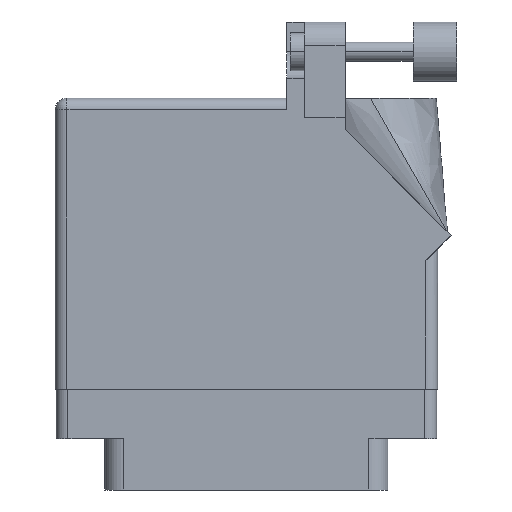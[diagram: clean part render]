
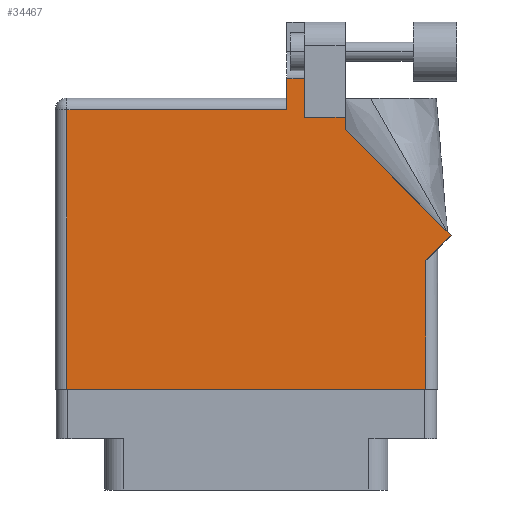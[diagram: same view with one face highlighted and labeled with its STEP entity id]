
A CAD part, front view. The second image highlights one B-rep face of the part: STEP entity #34467.
In plain terms, the highlighted face is planar.
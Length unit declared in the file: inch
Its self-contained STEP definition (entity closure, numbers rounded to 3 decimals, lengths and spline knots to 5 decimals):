
#255 = VECTOR ( 'NONE', #7287, 39.37008 ) ;
#1257 = VERTEX_POINT ( 'NONE', #19665 ) ;
#1385 = VECTOR ( 'NONE', #22672, 39.37008 ) ;
#1567 = LINE ( 'NONE', #26114, #7909 ) ;
#1798 = VERTEX_POINT ( 'NONE', #22263 ) ;
#2191 = CARTESIAN_POINT ( 'NONE',  ( 1.524, 1.36442, 0. ) ) ;
#2222 = LINE ( 'NONE', #28144, #1385 ) ;
#2418 = LINE ( 'NONE', #13033, #13001 ) ;
#2590 = VECTOR ( 'NONE', #5497, 39.37008 ) ;
#2717 = CARTESIAN_POINT ( 'NONE',  ( 1.948, 0.737, 0. ) ) ;
#2965 = VERTEX_POINT ( 'NONE', #5705 ) ;
#3114 = AXIS2_PLACEMENT_3D ( 'NONE', #13466, #18957, #32597 ) ;
#3211 = VERTEX_POINT ( 'NONE', #22888 ) ;
#4034 = DIRECTION ( 'NONE',  ( 0., 1., 0. ) ) ;
#5241 = EDGE_CURVE ( 'NONE', #28730, #2965, #20083, .T. ) ;
#5497 = DIRECTION ( 'NONE',  ( 1., 0., 0. ) ) ;
#5705 = CARTESIAN_POINT ( 'NONE',  ( 1.948, 0., 0. ) ) ;
#6089 = ORIENTED_EDGE ( 'NONE', *, *, #28696, .T. ) ;
#7287 = DIRECTION ( 'NONE',  ( 0., 1., 0. ) ) ;
#7909 = VECTOR ( 'NONE', #4034, 39.37008 ) ;
#8691 = EDGE_CURVE ( 'NONE', #3211, #1798, #18629, .T. ) ;
#8774 = DIRECTION ( 'NONE',  ( -1., 0., 0. ) ) ;
#8823 = EDGE_CURVE ( 'NONE', #13639, #29951, #1567, .T. ) ;
#9068 = ORIENTED_EDGE ( 'NONE', *, *, #5241, .T. ) ;
#9640 = ORIENTED_EDGE ( 'NONE', *, *, #9676, .T. ) ;
#9676 = EDGE_CURVE ( 'NONE', #1798, #28730, #2418, .T. ) ;
#10128 = EDGE_LOOP ( 'NONE', ( #23997, #32514, #20577, #15346, #9640, #9068, #22942, #32574, #21811, #6089, #27117 ) ) ;
#10708 = EDGE_CURVE ( 'NONE', #15570, #1257, #27729, .T. ) ;
#10904 = LINE ( 'NONE', #2191, #255 ) ;
#12149 = DIRECTION ( 'NONE',  ( -0.707, 0.707, 0. ) ) ;
#12798 = VECTOR ( 'NONE', #23317, 39.37008 ) ;
#13001 = VECTOR ( 'NONE', #32050, 39.37008 ) ;
#13033 = CARTESIAN_POINT ( 'NONE',  ( 0.062, 0., 0. ) ) ;
#13466 = CARTESIAN_POINT ( 'NONE',  ( 0., 1.53, 0. ) ) ;
#13639 = VERTEX_POINT ( 'NONE', #15105 ) ;
#14766 = CARTESIAN_POINT ( 'NONE',  ( 1.311, 1.6315, 0. ) ) ;
#14802 = CARTESIAN_POINT ( 'NONE',  ( 1.217, 1.53, 0. ) ) ;
#15105 = CARTESIAN_POINT ( 'NONE',  ( 1.311, 1.43, 0. ) ) ;
#15196 = EDGE_CURVE ( 'NONE', #29951, #26422, #27472, .T. ) ;
#15304 = CARTESIAN_POINT ( 'NONE',  ( 1.524, 1.43, 0. ) ) ;
#15346 = ORIENTED_EDGE ( 'NONE', *, *, #8691, .T. ) ;
#15507 = CARTESIAN_POINT ( 'NONE',  ( 0.062, 0., 0. ) ) ;
#15568 = EDGE_CURVE ( 'NONE', #33838, #13639, #29914, .T. ) ;
#15570 = VERTEX_POINT ( 'NONE', #18388 ) ;
#16088 = EDGE_CURVE ( 'NONE', #24751, #15570, #2222, .T. ) ;
#16403 = CARTESIAN_POINT ( 'NONE',  ( 1.64177, 1.6315, 0. ) ) ;
#16776 = VECTOR ( 'NONE', #30076, 39.37008 ) ;
#17356 = EDGE_CURVE ( 'NONE', #26422, #3211, #29828, .T. ) ;
#17864 = VECTOR ( 'NONE', #18813, 39.37008 ) ;
#18223 = EDGE_CURVE ( 'NONE', #2965, #24751, #25562, .T. ) ;
#18388 = CARTESIAN_POINT ( 'NONE',  ( 2.08071, 0.80771, 0. ) ) ;
#18629 = LINE ( 'NONE', #25144, #26313 ) ;
#18813 = DIRECTION ( 'NONE',  ( 0., 1., 0. ) ) ;
#18957 = DIRECTION ( 'NONE',  ( 0., 0., -1. ) ) ;
#19609 = VECTOR ( 'NONE', #12149, 39.37008 ) ;
#19665 = CARTESIAN_POINT ( 'NONE',  ( 1.524, 1.36442, 0. ) ) ;
#20083 = LINE ( 'NONE', #29794, #2590 ) ;
#20310 = CARTESIAN_POINT ( 'NONE',  ( 1.524, 1.43, 0. ) ) ;
#20577 = ORIENTED_EDGE ( 'NONE', *, *, #17356, .T. ) ;
#21139 = FACE_OUTER_BOUND ( 'NONE', #10128, .T. ) ;
#21811 = ORIENTED_EDGE ( 'NONE', *, *, #10708, .T. ) ;
#22263 = CARTESIAN_POINT ( 'NONE',  ( 0.062, 1.468, 0. ) ) ;
#22672 = DIRECTION ( 'NONE',  ( 0.707, 0.707, 0. ) ) ;
#22724 = VECTOR ( 'NONE', #34649, 39.37008 ) ;
#22888 = CARTESIAN_POINT ( 'NONE',  ( 1.217, 1.468, 0. ) ) ;
#22942 = ORIENTED_EDGE ( 'NONE', *, *, #18223, .T. ) ;
#23317 = DIRECTION ( 'NONE',  ( 0., -1., 0. ) ) ;
#23997 = ORIENTED_EDGE ( 'NONE', *, *, #8823, .T. ) ;
#24751 = VERTEX_POINT ( 'NONE', #35174 ) ;
#25144 = CARTESIAN_POINT ( 'NONE',  ( 0., 1.468, 0. ) ) ;
#25562 = LINE ( 'NONE', #2717, #17864 ) ;
#25757 = CARTESIAN_POINT ( 'NONE',  ( 2.08071, 0.80771, 0. ) ) ;
#26114 = CARTESIAN_POINT ( 'NONE',  ( 1.311, 1.43, 0. ) ) ;
#26313 = VECTOR ( 'NONE', #8774, 39.37008 ) ;
#26422 = VERTEX_POINT ( 'NONE', #35077 ) ;
#27117 = ORIENTED_EDGE ( 'NONE', *, *, #15568, .T. ) ;
#27472 = LINE ( 'NONE', #16403, #16776 ) ;
#27729 = LINE ( 'NONE', #25757, #19609 ) ;
#28144 = CARTESIAN_POINT ( 'NONE',  ( 2.01, 0.737, 0. ) ) ;
#28696 = EDGE_CURVE ( 'NONE', #1257, #33838, #10904, .T. ) ;
#28730 = VERTEX_POINT ( 'NONE', #15507 ) ;
#29794 = CARTESIAN_POINT ( 'NONE',  ( 0., 0., 0. ) ) ;
#29828 = LINE ( 'NONE', #14802, #12798 ) ;
#29914 = LINE ( 'NONE', #20310, #22724 ) ;
#29951 = VERTEX_POINT ( 'NONE', #14766 ) ;
#30076 = DIRECTION ( 'NONE',  ( -1., 0., 0. ) ) ;
#32050 = DIRECTION ( 'NONE',  ( 0., -1., 0. ) ) ;
#32253 = PLANE ( 'NONE',  #3114 ) ;
#32514 = ORIENTED_EDGE ( 'NONE', *, *, #15196, .T. ) ;
#32574 = ORIENTED_EDGE ( 'NONE', *, *, #16088, .T. ) ;
#32597 = DIRECTION ( 'NONE',  ( -1., 0., 0. ) ) ;
#33838 = VERTEX_POINT ( 'NONE', #15304 ) ;
#34467 = ADVANCED_FACE ( 'NONE', ( #21139 ), #32253, .F. ) ;
#34649 = DIRECTION ( 'NONE',  ( -1., 0., 0. ) ) ;
#35077 = CARTESIAN_POINT ( 'NONE',  ( 1.217, 1.6315, 0. ) ) ;
#35174 = CARTESIAN_POINT ( 'NONE',  ( 1.948, 0.675, 0. ) ) ;
